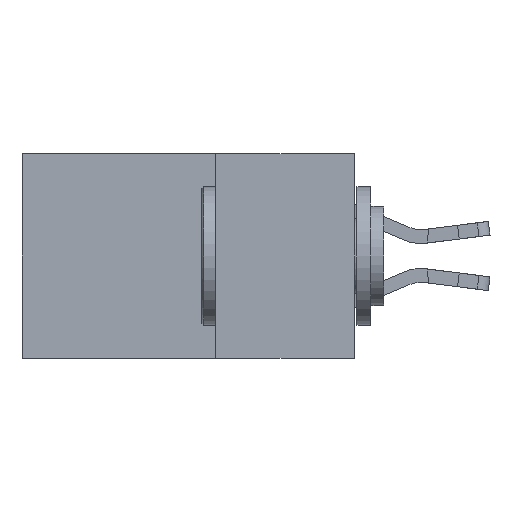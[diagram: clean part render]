
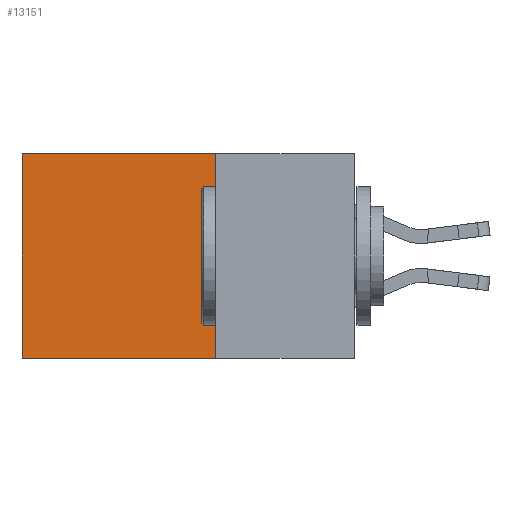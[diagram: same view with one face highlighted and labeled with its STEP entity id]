
A CAD part, left-side view. The second image highlights one B-rep face of the part: STEP entity #13151.
In plain terms, the highlighted planar face has unit normal (-1, 0, 0).
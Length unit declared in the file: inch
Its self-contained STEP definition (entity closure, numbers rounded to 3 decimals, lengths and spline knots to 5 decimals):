
#469 = EDGE_LOOP ( 'NONE', ( #16623, #10098, #1443, #1885 ) ) ;
#680 = CARTESIAN_POINT ( 'NONE',  ( 0.298, 0.25, 0. ) ) ;
#888 = VECTOR ( 'NONE', #19176, 39.37008 ) ;
#1104 = DIRECTION ( 'NONE',  ( 0., 1., 0. ) ) ;
#1409 = CARTESIAN_POINT ( 'NONE',  ( 0.298, 0.6, -0.37 ) ) ;
#1443 = ORIENTED_EDGE ( 'NONE', *, *, #2414, .F. ) ;
#1766 = FACE_OUTER_BOUND ( 'NONE', #469, .T. ) ;
#1885 = ORIENTED_EDGE ( 'NONE', *, *, #8029, .T. ) ;
#2215 = CARTESIAN_POINT ( 'NONE',  ( 0.298, 0.6, 0. ) ) ;
#2414 = EDGE_CURVE ( 'NONE', #15399, #24826, #6311, .T. ) ;
#3125 = CARTESIAN_POINT ( 'NONE',  ( 0.298, 0.6, 0. ) ) ;
#3609 = LINE ( 'NONE', #7154, #18018 ) ;
#5240 = VECTOR ( 'NONE', #18793, 39.37008 ) ;
#6311 = LINE ( 'NONE', #680, #888 ) ;
#6501 = VECTOR ( 'NONE', #1104, 39.37008 ) ;
#7154 = CARTESIAN_POINT ( 'NONE',  ( 0.298, 0.25, -0.37 ) ) ;
#7385 = CARTESIAN_POINT ( 'NONE',  ( 0.298, 0.25, 0. ) ) ;
#8029 = EDGE_CURVE ( 'NONE', #15399, #17492, #12397, .T. ) ;
#9236 = EDGE_CURVE ( 'NONE', #17492, #11826, #11161, .T. ) ;
#9413 = PLANE ( 'NONE',  #21600 ) ;
#10098 = ORIENTED_EDGE ( 'NONE', *, *, #14680, .F. ) ;
#11161 = LINE ( 'NONE', #3125, #5240 ) ;
#11361 = DIRECTION ( 'NONE',  ( 0., 0., -1. ) ) ;
#11826 = VERTEX_POINT ( 'NONE', #1409 ) ;
#12397 = LINE ( 'NONE', #18846, #6501 ) ;
#13087 = DIRECTION ( 'NONE',  ( 0., 1., 0. ) ) ;
#13151 = ADVANCED_FACE ( 'NONE', ( #1766 ), #9413, .F. ) ;
#14680 = EDGE_CURVE ( 'NONE', #24826, #11826, #3609, .T. ) ;
#15399 = VERTEX_POINT ( 'NONE', #22726 ) ;
#16623 = ORIENTED_EDGE ( 'NONE', *, *, #9236, .T. ) ;
#17492 = VERTEX_POINT ( 'NONE', #2215 ) ;
#18018 = VECTOR ( 'NONE', #13087, 39.37008 ) ;
#18793 = DIRECTION ( 'NONE',  ( 0., 0., -1. ) ) ;
#18846 = CARTESIAN_POINT ( 'NONE',  ( 0.298, 0.25, 0. ) ) ;
#19176 = DIRECTION ( 'NONE',  ( 0., 0., -1. ) ) ;
#20790 = CARTESIAN_POINT ( 'NONE',  ( 0.298, 0.25, -0.37 ) ) ;
#21600 = AXIS2_PLACEMENT_3D ( 'NONE', #7385, #22718, #11361 ) ;
#22718 = DIRECTION ( 'NONE',  ( 1., 0., 0. ) ) ;
#22726 = CARTESIAN_POINT ( 'NONE',  ( 0.298, 0.25, 0. ) ) ;
#24826 = VERTEX_POINT ( 'NONE', #20790 ) ;
